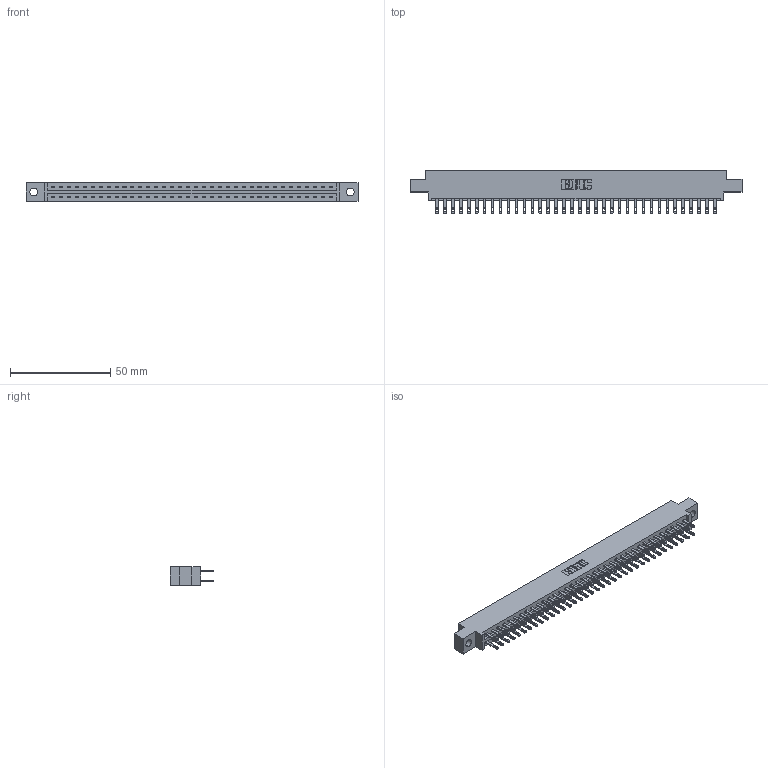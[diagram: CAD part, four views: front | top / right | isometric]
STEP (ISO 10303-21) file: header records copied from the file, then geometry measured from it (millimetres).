
FILE_DESCRIPTION (( 'STEP AP203' ), '1' );
FILE_NAME ('337-072-500-804.STEP', '2018-08-11T13:46:04', ( '' ), ( '' ), 'SwSTEP 2.0', 'SolidWorks 2016', '' );
FILE_SCHEMA (( 'CONFIG_CONTROL_DESIGN' ));
Length unit declared in the file: inch
Products named in the file (3): 337 Part_0.170 Offset - 0.156 Dia-TH; 345-292-001_345-293-100; 337-072-500-804
Assembly tree (73 placements, depth 2):
  337-072-500-804
    337 Part_0.170 Offset - 0.156 Dia-TH
    345-292-001_345-293-100  x72
Bounding box: 165.66 x 21.85 x 9.4 mm (x, y, z)
Volume: 17393.2 mm3; surface area: 20308.9 mm2
Topology: 73 solids, 73 shells, 3718 faces, 11339 edges, 7558 vertices
Faces by surface type: plane 2378, cylinder 1340
Entity records: 28753 total; most frequent: CARTESIAN_POINT 4850, ORIENTED_EDGE 4786, DIRECTION 4137, EDGE_CURVE 2393, VECTOR 2261, LINE 2261, VERTEX_POINT 1594, AXIS2_PLACEMENT_3D 938
